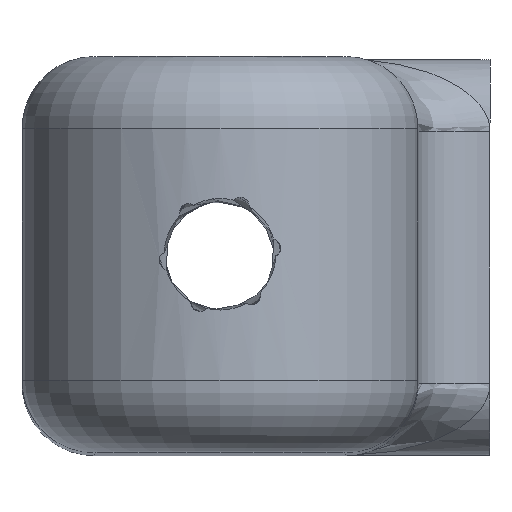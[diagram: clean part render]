
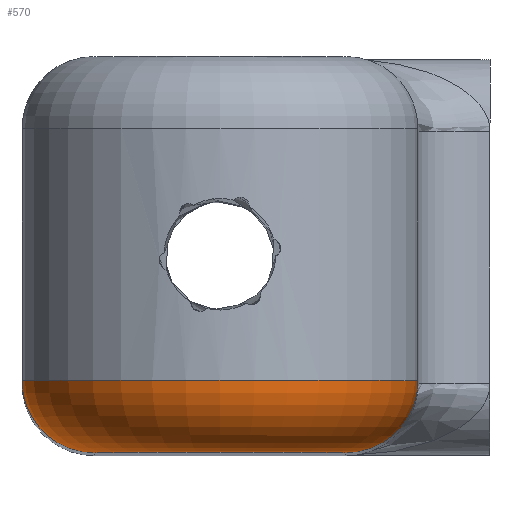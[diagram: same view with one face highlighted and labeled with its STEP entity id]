
A CAD part, top view. The second image highlights one B-rep face of the part: STEP entity #570.
In plain terms, the highlighted toroidal (fillet/blend) face has major radius 7 mm and minor radius 4 mm.
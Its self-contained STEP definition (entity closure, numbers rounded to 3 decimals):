
#238=CARTESIAN_POINT('',(11.,-7.,99.0));
#239=VERTEX_POINT('',#238);
#246=CARTESIAN_POINT('',(7.,-11.0,99.0));
#247=VERTEX_POINT('',#246);
#248=CARTESIAN_POINT('',(7.,-7.,99.0));
#249=DIRECTION('',(0.0,0.0,1.0));
#250=DIRECTION('',(0.0,-1.0,0.0));
#251=AXIS2_PLACEMENT_3D('',#248,#249,#250);
#252=CIRCLE('',#251,4.0);
#253=EDGE_CURVE('',#247,#239,#252,.T.);
#474=CARTESIAN_POINT('',(-11.,-7.,99.0));
#475=VERTEX_POINT('',#474);
#505=CARTESIAN_POINT('',(-7.,-11.0,99.0));
#506=VERTEX_POINT('',#505);
#513=CARTESIAN_POINT('',(-7.,-7.,99.0));
#514=DIRECTION('',(0.0,0.0,-1.0));
#515=DIRECTION('',(0.0,-1.0,0.0));
#516=AXIS2_PLACEMENT_3D('',#513,#514,#515);
#517=CIRCLE('',#516,4.0);
#518=EDGE_CURVE('',#506,#475,#517,.T.);
#547=CARTESIAN_POINT('',(0.,-7.,99.0));
#548=DIRECTION('',(0.0,1.0,0.0));
#549=DIRECTION('',(0.0,0.0,1.0));
#550=AXIS2_PLACEMENT_3D('',#547,#548,#549);
#551=TOROIDAL_SURFACE('',#550,7.,4.0);
#552=ORIENTED_EDGE('',*,*,#253,.T.);
#553=CARTESIAN_POINT('',(0.,-7.,99.0));
#554=DIRECTION('',(0.0,-1.0,0.0));
#555=DIRECTION('',(0.0,0.0,1.0));
#556=AXIS2_PLACEMENT_3D('',#553,#554,#555);
#557=CIRCLE('',#556,11.0);
#558=EDGE_CURVE('',#239,#475,#557,.T.);
#559=ORIENTED_EDGE('',*,*,#558,.T.);
#560=ORIENTED_EDGE('',*,*,#518,.F.);
#561=CARTESIAN_POINT('',(0.,-11.0,99.0));
#562=DIRECTION('',(0.0,1.0,0.0));
#563=DIRECTION('',(0.0,0.0,1.0));
#564=AXIS2_PLACEMENT_3D('',#561,#562,#563);
#565=CIRCLE('',#564,7.);
#566=EDGE_CURVE('',#506,#247,#565,.T.);
#567=ORIENTED_EDGE('',*,*,#566,.T.);
#568=EDGE_LOOP('',(#552,#559,#560,#567));
#569=FACE_OUTER_BOUND('',#568,.T.);
#570=ADVANCED_FACE('',(#569),#551,.T.);
